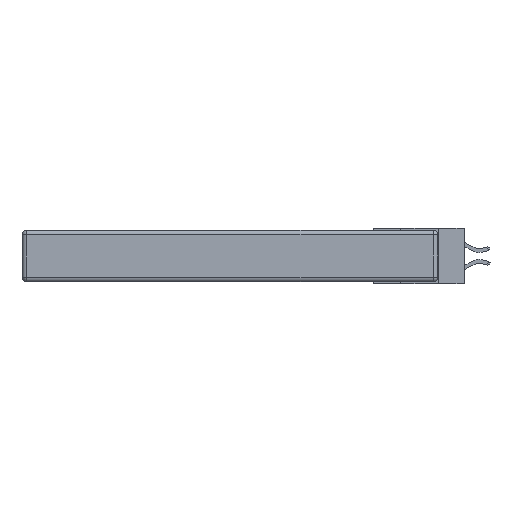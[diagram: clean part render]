
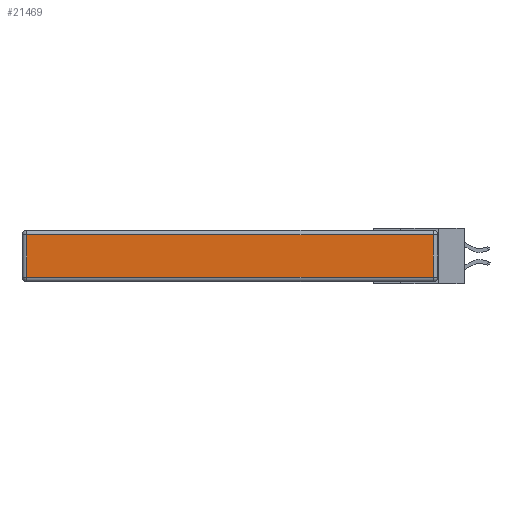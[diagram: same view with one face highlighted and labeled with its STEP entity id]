
A CAD part, left-side view. The second image highlights one B-rep face of the part: STEP entity #21469.
In plain terms, the highlighted planar face has unit normal (-1, 0, 0).
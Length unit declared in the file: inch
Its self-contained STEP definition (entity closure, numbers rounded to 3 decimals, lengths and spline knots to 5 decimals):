
#15 = FACE_OUTER_BOUND ( 'NONE', #41, .T. ) ;
#41 = EDGE_LOOP ( 'NONE', ( #20239, #20256, #14160, #19058 ) ) ;
#174 = CARTESIAN_POINT ( 'NONE',  ( 0., 0.03, -0.343 ) ) ;
#415 = DIRECTION ( 'NONE',  ( 0., 0., 1. ) ) ;
#525 = EDGE_CURVE ( 'NONE', #6943, #16445, #18639, .T. ) ;
#1895 = VECTOR ( 'NONE', #10031, 39.37008 ) ;
#2627 = VECTOR ( 'NONE', #12875, 39.37008 ) ;
#3611 = VERTEX_POINT ( 'NONE', #4794 ) ;
#4794 = CARTESIAN_POINT ( 'NONE',  ( 0., 0.03, -0.313 ) ) ;
#6943 = VERTEX_POINT ( 'NONE', #15218 ) ;
#7104 = DIRECTION ( 'NONE',  ( -1., 0., 0. ) ) ;
#7317 = CARTESIAN_POINT ( 'NONE',  ( 0., 2.72, -0.313 ) ) ;
#7968 = EDGE_CURVE ( 'NONE', #16885, #3611, #19557, .T. ) ;
#7979 = EDGE_CURVE ( 'NONE', #3611, #6943, #17445, .T. ) ;
#9398 = CARTESIAN_POINT ( 'NONE',  ( 0., 2.72, -0.03 ) ) ;
#9624 = CARTESIAN_POINT ( 'NONE',  ( 0., 2.72, -0.343 ) ) ;
#9677 = VECTOR ( 'NONE', #13412, 39.37008 ) ;
#10031 = DIRECTION ( 'NONE',  ( 0., -1., 0. ) ) ;
#12059 = CARTESIAN_POINT ( 'NONE',  ( 0., 0., -0.343 ) ) ;
#12875 = DIRECTION ( 'NONE',  ( 0., 0., -1. ) ) ;
#13412 = DIRECTION ( 'NONE',  ( 0., 0., 1. ) ) ;
#14160 = ORIENTED_EDGE ( 'NONE', *, *, #525, .T. ) ;
#15187 = CARTESIAN_POINT ( 'NONE',  ( 0., 2.75, -0.03 ) ) ;
#15218 = CARTESIAN_POINT ( 'NONE',  ( 0., 0.03, -0.03 ) ) ;
#16445 = VERTEX_POINT ( 'NONE', #9398 ) ;
#16885 = VERTEX_POINT ( 'NONE', #7317 ) ;
#17056 = AXIS2_PLACEMENT_3D ( 'NONE', #12059, #7104, #415 ) ;
#17445 = LINE ( 'NONE', #174, #9677 ) ;
#18536 = CARTESIAN_POINT ( 'NONE',  ( 0., 0., -0.313 ) ) ;
#18553 = PLANE ( 'NONE',  #17056 ) ;
#18639 = LINE ( 'NONE', #15187, #19930 ) ;
#19058 = ORIENTED_EDGE ( 'NONE', *, *, #21226, .T. ) ;
#19557 = LINE ( 'NONE', #18536, #1895 ) ;
#19750 = LINE ( 'NONE', #9624, #2627 ) ;
#19930 = VECTOR ( 'NONE', #20077, 39.37008 ) ;
#20077 = DIRECTION ( 'NONE',  ( 0., 1., 0. ) ) ;
#20239 = ORIENTED_EDGE ( 'NONE', *, *, #7968, .T. ) ;
#20256 = ORIENTED_EDGE ( 'NONE', *, *, #7979, .T. ) ;
#21226 = EDGE_CURVE ( 'NONE', #16445, #16885, #19750, .T. ) ;
#21469 = ADVANCED_FACE ( 'NONE', ( #15 ), #18553, .T. ) ;
